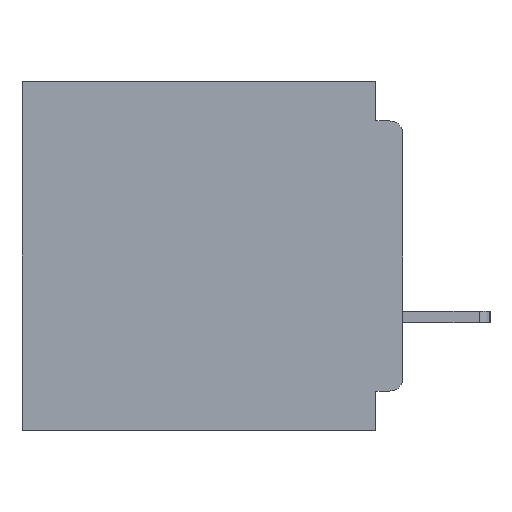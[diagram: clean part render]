
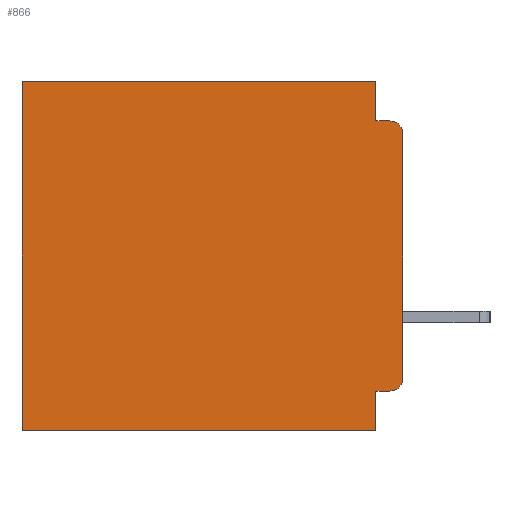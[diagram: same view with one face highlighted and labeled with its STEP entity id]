
A CAD part, left-side view. The second image highlights one B-rep face of the part: STEP entity #866.
In plain terms, the highlighted planar face has unit normal (-1, 0, 0).
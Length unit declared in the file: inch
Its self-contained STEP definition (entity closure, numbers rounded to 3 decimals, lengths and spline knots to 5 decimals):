
#441 = EDGE_CURVE ( 'NONE', #13946, #21190, #40193, .T. ) ;
#507 = DIRECTION ( 'NONE',  ( 0., 0., -1. ) ) ;
#853 = LINE ( 'NONE', #24819, #8679 ) ;
#866 = ADVANCED_FACE ( 'NONE', ( #3868 ), #30303, .F. ) ;
#2396 = DIRECTION ( 'NONE',  ( 0., 0., -1. ) ) ;
#2526 = VECTOR ( 'NONE', #38475, 39.37008 ) ;
#3868 = FACE_OUTER_BOUND ( 'NONE', #6932, .T. ) ;
#4364 = CARTESIAN_POINT ( 'NONE',  ( 0.3, 0.031, -0.4 ) ) ;
#4784 = EDGE_CURVE ( 'NONE', #18921, #19405, #40792, .T. ) ;
#4906 = VERTEX_POINT ( 'NONE', #39871 ) ;
#5335 = CARTESIAN_POINT ( 'NONE',  ( 0.3, 0., -0.045 ) ) ;
#5956 = CARTESIAN_POINT ( 'NONE',  ( 0.3, 0.015, -0.355 ) ) ;
#6932 = EDGE_LOOP ( 'NONE', ( #41456, #12386, #23196, #23849, #40963, #18946, #31100, #37105, #10811, #18127 ) ) ;
#7462 = LINE ( 'NONE', #5335, #41587 ) ;
#7878 = CARTESIAN_POINT ( 'NONE',  ( 0.3, 0., -0.4 ) ) ;
#8228 = CARTESIAN_POINT ( 'NONE',  ( 0.3, 0.031, -0.355 ) ) ;
#8320 = CARTESIAN_POINT ( 'NONE',  ( 0.3, 0.437, -0.4 ) ) ;
#8331 = DIRECTION ( 'NONE',  ( 0., 1., 0. ) ) ;
#8679 = VECTOR ( 'NONE', #8331, 39.37008 ) ;
#9121 = AXIS2_PLACEMENT_3D ( 'NONE', #19225, #42377, #22569 ) ;
#9368 = DIRECTION ( 'NONE',  ( -1., 0., 0. ) ) ;
#10581 = CARTESIAN_POINT ( 'NONE',  ( 0.3, 0., -0.06 ) ) ;
#10811 = ORIENTED_EDGE ( 'NONE', *, *, #441, .F. ) ;
#11977 = DIRECTION ( 'NONE',  ( 0., -1., 0. ) ) ;
#12139 = LINE ( 'NONE', #33575, #27695 ) ;
#12375 = CIRCLE ( 'NONE', #9121, 0.015 ) ;
#12386 = ORIENTED_EDGE ( 'NONE', *, *, #40425, .T. ) ;
#13676 = EDGE_CURVE ( 'NONE', #4906, #19405, #39149, .T. ) ;
#13806 = VECTOR ( 'NONE', #27677, 39.37008 ) ;
#13843 = AXIS2_PLACEMENT_3D ( 'NONE', #29185, #9368, #32538 ) ;
#13946 = VERTEX_POINT ( 'NONE', #5956 ) ;
#16410 = CIRCLE ( 'NONE', #13843, 0.015 ) ;
#17159 = EDGE_CURVE ( 'NONE', #31742, #18921, #853, .T. ) ;
#17614 = CARTESIAN_POINT ( 'NONE',  ( 0.3, 0., -0.34 ) ) ;
#18083 = VERTEX_POINT ( 'NONE', #10581 ) ;
#18127 = ORIENTED_EDGE ( 'NONE', *, *, #35162, .T. ) ;
#18614 = EDGE_CURVE ( 'NONE', #31742, #35683, #12139, .T. ) ;
#18839 = AXIS2_PLACEMENT_3D ( 'NONE', #22068, #21590, #2396 ) ;
#18921 = VERTEX_POINT ( 'NONE', #38689 ) ;
#18946 = ORIENTED_EDGE ( 'NONE', *, *, #4784, .T. ) ;
#19225 = CARTESIAN_POINT ( 'NONE',  ( 0.3, 0.015, -0.06 ) ) ;
#19385 = DIRECTION ( 'NONE',  ( 0., 0., -1. ) ) ;
#19405 = VERTEX_POINT ( 'NONE', #8320 ) ;
#21190 = VERTEX_POINT ( 'NONE', #8228 ) ;
#21199 = LINE ( 'NONE', #38333, #2526 ) ;
#21468 = CARTESIAN_POINT ( 'NONE',  ( 0.3, 0.437, -0.4 ) ) ;
#21590 = DIRECTION ( 'NONE',  ( 1., 0., 0. ) ) ;
#22068 = CARTESIAN_POINT ( 'NONE',  ( 0.3, 0., -0.4 ) ) ;
#22569 = DIRECTION ( 'NONE',  ( 0., 0., -1. ) ) ;
#22631 = CARTESIAN_POINT ( 'NONE',  ( 0.3, 0., -0.355 ) ) ;
#23196 = ORIENTED_EDGE ( 'NONE', *, *, #30995, .F. ) ;
#23849 = ORIENTED_EDGE ( 'NONE', *, *, #18614, .F. ) ;
#24320 = DIRECTION ( 'NONE',  ( 0., 1., 0. ) ) ;
#24819 = CARTESIAN_POINT ( 'NONE',  ( 0.3, 0., 0. ) ) ;
#25242 = VECTOR ( 'NONE', #30877, 39.37008 ) ;
#25379 = CARTESIAN_POINT ( 'NONE',  ( 0.3, 0.015, -0.045 ) ) ;
#27677 = DIRECTION ( 'NONE',  ( 0., 1., 0. ) ) ;
#27695 = VECTOR ( 'NONE', #507, 39.37008 ) ;
#29185 = CARTESIAN_POINT ( 'NONE',  ( 0.3, 0.015, -0.34 ) ) ;
#30303 = PLANE ( 'NONE',  #18839 ) ;
#30877 = DIRECTION ( 'NONE',  ( 0., 0., -1. ) ) ;
#30995 = EDGE_CURVE ( 'NONE', #35683, #41709, #7462, .T. ) ;
#31100 = ORIENTED_EDGE ( 'NONE', *, *, #13676, .F. ) ;
#31742 = VERTEX_POINT ( 'NONE', #35652 ) ;
#32538 = DIRECTION ( 'NONE',  ( 0., 0., -1. ) ) ;
#32645 = EDGE_CURVE ( 'NONE', #18083, #42599, #21199, .T. ) ;
#33575 = CARTESIAN_POINT ( 'NONE',  ( 0.3, 0.031, 0. ) ) ;
#34062 = LINE ( 'NONE', #4364, #25242 ) ;
#34208 = EDGE_CURVE ( 'NONE', #21190, #4906, #34062, .T. ) ;
#35162 = EDGE_CURVE ( 'NONE', #13946, #42599, #16410, .T. ) ;
#35652 = CARTESIAN_POINT ( 'NONE',  ( 0.3, 0.031, 0. ) ) ;
#35683 = VERTEX_POINT ( 'NONE', #36671 ) ;
#36671 = CARTESIAN_POINT ( 'NONE',  ( 0.3, 0.031, -0.045 ) ) ;
#37105 = ORIENTED_EDGE ( 'NONE', *, *, #34208, .F. ) ;
#38064 = VECTOR ( 'NONE', #24320, 39.37008 ) ;
#38333 = CARTESIAN_POINT ( 'NONE',  ( 0.3, 0., -0.4 ) ) ;
#38475 = DIRECTION ( 'NONE',  ( 0., 0., -1. ) ) ;
#38689 = CARTESIAN_POINT ( 'NONE',  ( 0.3, 0.437, 0. ) ) ;
#39149 = LINE ( 'NONE', #7878, #13806 ) ;
#39765 = VECTOR ( 'NONE', #19385, 39.37008 ) ;
#39871 = CARTESIAN_POINT ( 'NONE',  ( 0.3, 0.031, -0.4 ) ) ;
#40193 = LINE ( 'NONE', #22631, #38064 ) ;
#40425 = EDGE_CURVE ( 'NONE', #18083, #41709, #12375, .T. ) ;
#40792 = LINE ( 'NONE', #21468, #39765 ) ;
#40963 = ORIENTED_EDGE ( 'NONE', *, *, #17159, .T. ) ;
#41456 = ORIENTED_EDGE ( 'NONE', *, *, #32645, .F. ) ;
#41587 = VECTOR ( 'NONE', #11977, 39.37008 ) ;
#41709 = VERTEX_POINT ( 'NONE', #25379 ) ;
#42377 = DIRECTION ( 'NONE',  ( -1., 0., 0. ) ) ;
#42599 = VERTEX_POINT ( 'NONE', #17614 ) ;
